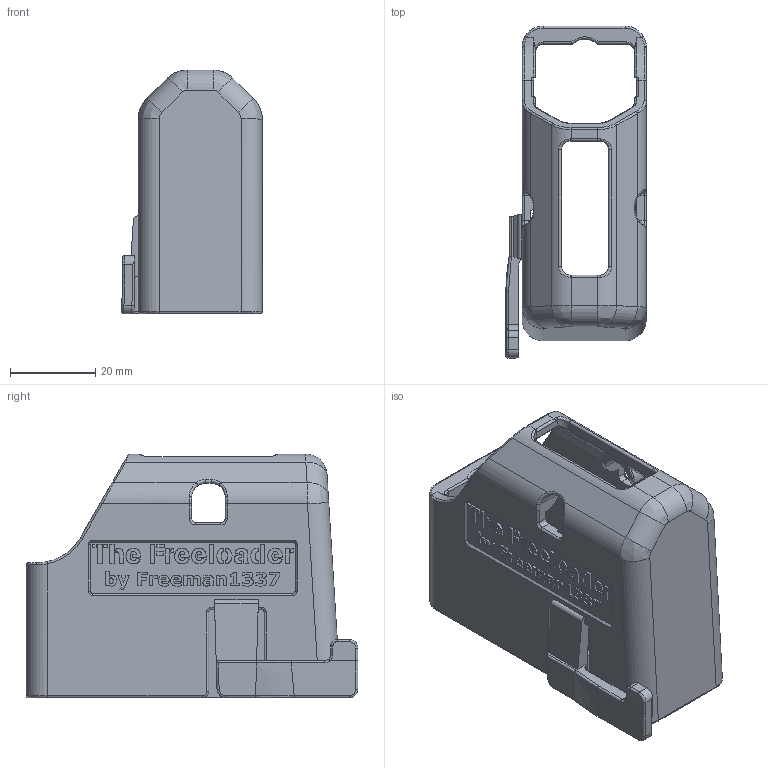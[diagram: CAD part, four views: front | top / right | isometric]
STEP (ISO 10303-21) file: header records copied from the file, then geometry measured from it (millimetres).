
FILE_DESCRIPTION(/* description */ (''),/* implementation_level */ '2;1');
FILE_NAME(/* name */ 'freeloader-body-intergrated-magcatch-engraved-v6.step',/* time_stamp */ '2021-09-20T14:46:06-07:00',/* author */ (''),/* organization */ (''),/* preprocessor_version */ 'ST-DEVELOPER v18.1',/* originating_system */ 'Autodesk Translation Framework v10.10.0.1391',/* authorisation */ '');
FILE_SCHEMA (('AUTOMOTIVE_DESIGN { 1 0 10303 214 3 1 1 }'));
Products named in the file (1): loader-base-v2-useThis
Bounding box: 33.05 x 78 x 57.31 mm (x, y, z)
Volume: 28370.8 mm3; surface area: 21297.4 mm2
Topology: 1 solids, 1 shells, 2444 faces, 6656 edges, 4374 vertices
Faces by surface type: bspline 1528, plane 725, cylinder 142, torus 45, cone 4
Entity records: 86783 total; most frequent: CARTESIAN_POINT 37074, ORIENTED_EDGE 13306, EDGE_CURVE 6653, DIRECTION 6368, VERTEX_POINT 4374, LINE 3174, VECTOR 3174, EDGE_LOOP 2615
